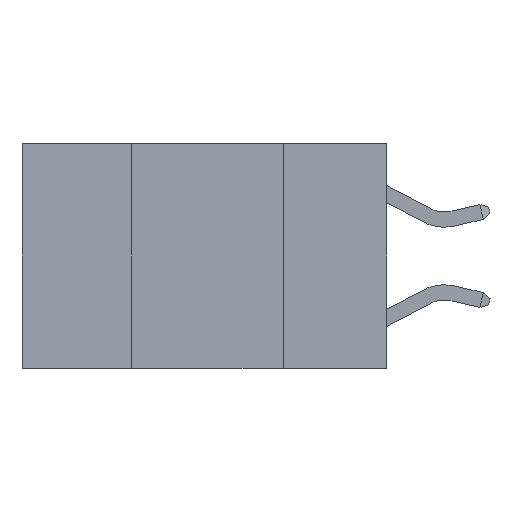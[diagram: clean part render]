
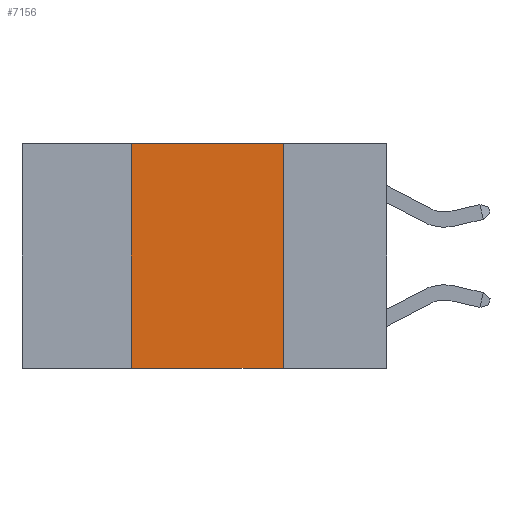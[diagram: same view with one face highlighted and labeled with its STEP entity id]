
A CAD part, left-side view. The second image highlights one B-rep face of the part: STEP entity #7156.
In plain terms, the highlighted planar face has unit normal (-1, 0, 0).
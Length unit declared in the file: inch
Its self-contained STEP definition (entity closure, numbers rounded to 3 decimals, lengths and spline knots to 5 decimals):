
#72 = LINE ( 'NONE', #6864, #5147 ) ;
#124 = VERTEX_POINT ( 'NONE', #6790 ) ;
#355 = EDGE_LOOP ( 'NONE', ( #9569, #7437, #10529, #511 ) ) ;
#511 = ORIENTED_EDGE ( 'NONE', *, *, #10780, .T. ) ;
#857 = DIRECTION ( 'NONE',  ( 0., 0., 1. ) ) ;
#913 = VERTEX_POINT ( 'NONE', #1603 ) ;
#1094 = FACE_OUTER_BOUND ( 'NONE', #355, .T. ) ;
#1352 = VECTOR ( 'NONE', #2093, 39.37008 ) ;
#1603 = CARTESIAN_POINT ( 'NONE',  ( 0., 0.17, -0.37 ) ) ;
#2093 = DIRECTION ( 'NONE',  ( 0., -1., 0. ) ) ;
#2479 = CARTESIAN_POINT ( 'NONE',  ( 0., 0.42, -0.37 ) ) ;
#2481 = VECTOR ( 'NONE', #12931, 39.37008 ) ;
#2586 = VERTEX_POINT ( 'NONE', #2479 ) ;
#5147 = VECTOR ( 'NONE', #11048, 39.37008 ) ;
#5325 = CARTESIAN_POINT ( 'NONE',  ( 0., 0.6, 0. ) ) ;
#5356 = LINE ( 'NONE', #7724, #2481 ) ;
#5557 = DIRECTION ( 'NONE',  ( 1., 0., 0. ) ) ;
#5601 = EDGE_CURVE ( 'NONE', #2586, #6164, #12624, .T. ) ;
#6164 = VERTEX_POINT ( 'NONE', #12391 ) ;
#6790 = CARTESIAN_POINT ( 'NONE',  ( 0., 0.17, 0. ) ) ;
#6864 = CARTESIAN_POINT ( 'NONE',  ( 0., 0.17, 0. ) ) ;
#7156 = ADVANCED_FACE ( 'NONE', ( #1094 ), #10806, .F. ) ;
#7437 = ORIENTED_EDGE ( 'NONE', *, *, #8298, .F. ) ;
#7724 = CARTESIAN_POINT ( 'NONE',  ( 0., 0.6, -0.37 ) ) ;
#8298 = EDGE_CURVE ( 'NONE', #6164, #124, #12540, .T. ) ;
#9197 = VECTOR ( 'NONE', #857, 39.37008 ) ;
#9438 = CARTESIAN_POINT ( 'NONE',  ( 0., 0.42, 0. ) ) ;
#9569 = ORIENTED_EDGE ( 'NONE', *, *, #13216, .F. ) ;
#9776 = CARTESIAN_POINT ( 'NONE',  ( 0., 0.6, 0. ) ) ;
#10462 = AXIS2_PLACEMENT_3D ( 'NONE', #9776, #5557, #12921 ) ;
#10529 = ORIENTED_EDGE ( 'NONE', *, *, #5601, .F. ) ;
#10780 = EDGE_CURVE ( 'NONE', #2586, #913, #5356, .T. ) ;
#10806 = PLANE ( 'NONE',  #10462 ) ;
#11048 = DIRECTION ( 'NONE',  ( 0., 0., -1. ) ) ;
#12391 = CARTESIAN_POINT ( 'NONE',  ( 0., 0.42, 0. ) ) ;
#12540 = LINE ( 'NONE', #5325, #1352 ) ;
#12624 = LINE ( 'NONE', #9438, #9197 ) ;
#12921 = DIRECTION ( 'NONE',  ( 0., 0., -1. ) ) ;
#12931 = DIRECTION ( 'NONE',  ( 0., -1., 0. ) ) ;
#13216 = EDGE_CURVE ( 'NONE', #124, #913, #72, .T. ) ;
